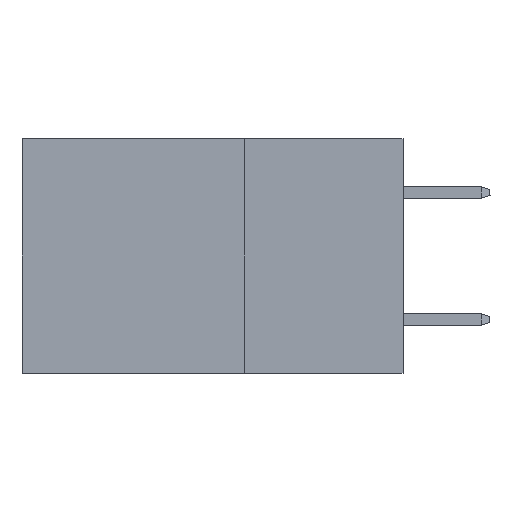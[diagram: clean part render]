
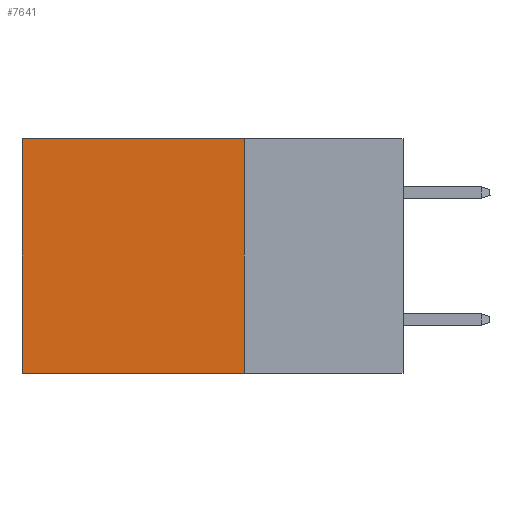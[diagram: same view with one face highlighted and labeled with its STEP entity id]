
A CAD part, left-side view. The second image highlights one B-rep face of the part: STEP entity #7641.
In plain terms, the highlighted planar face has unit normal (-1, 0, 0).
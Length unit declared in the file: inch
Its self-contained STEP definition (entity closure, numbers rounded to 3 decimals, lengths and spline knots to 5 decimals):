
#786 = DIRECTION ( 'NONE',  ( 1., 0., 0. ) ) ;
#1790 = CARTESIAN_POINT ( 'NONE',  ( 0.2875, 0.25, -0.37 ) ) ;
#4388 = DIRECTION ( 'NONE',  ( 0., 0., -1. ) ) ;
#4573 = DIRECTION ( 'NONE',  ( 0., 0., -1. ) ) ;
#4830 = CARTESIAN_POINT ( 'NONE',  ( 0.2875, 0.25, 0. ) ) ;
#6006 = ORIENTED_EDGE ( 'NONE', *, *, #22794, .F. ) ;
#7256 = VECTOR ( 'NONE', #27982, 39.37008 ) ;
#7554 = PLANE ( 'NONE',  #19619 ) ;
#7641 = ADVANCED_FACE ( 'NONE', ( #35799 ), #7554, .F. ) ;
#7996 = ORIENTED_EDGE ( 'NONE', *, *, #14541, .T. ) ;
#9535 = VECTOR ( 'NONE', #41426, 39.37008 ) ;
#10959 = CARTESIAN_POINT ( 'NONE',  ( 0.2875, 0.25, 0. ) ) ;
#13376 = CARTESIAN_POINT ( 'NONE',  ( 0.2875, 0.6, 0. ) ) ;
#14541 = EDGE_CURVE ( 'NONE', #29327, #15998, #15408, .T. ) ;
#15018 = VERTEX_POINT ( 'NONE', #1790 ) ;
#15116 = DIRECTION ( 'NONE',  ( 0., 0., -1. ) ) ;
#15408 = LINE ( 'NONE', #19041, #36087 ) ;
#15998 = VERTEX_POINT ( 'NONE', #42530 ) ;
#19041 = CARTESIAN_POINT ( 'NONE',  ( 0.2875, 0.6, 0. ) ) ;
#19619 = AXIS2_PLACEMENT_3D ( 'NONE', #4830, #786, #4388 ) ;
#21358 = LINE ( 'NONE', #27669, #9535 ) ;
#22794 = EDGE_CURVE ( 'NONE', #27226, #15018, #25311, .T. ) ;
#25311 = LINE ( 'NONE', #32509, #34199 ) ;
#27226 = VERTEX_POINT ( 'NONE', #10959 ) ;
#27669 = CARTESIAN_POINT ( 'NONE',  ( 0.2875, 0.25, -0.37 ) ) ;
#27982 = DIRECTION ( 'NONE',  ( 0., 1., 0. ) ) ;
#29327 = VERTEX_POINT ( 'NONE', #13376 ) ;
#30481 = CARTESIAN_POINT ( 'NONE',  ( 0.2875, 0.25, 0. ) ) ;
#32103 = EDGE_CURVE ( 'NONE', #27226, #29327, #44274, .T. ) ;
#32509 = CARTESIAN_POINT ( 'NONE',  ( 0.2875, 0.25, 0. ) ) ;
#34091 = EDGE_LOOP ( 'NONE', ( #7996, #34408, #6006, #35212 ) ) ;
#34199 = VECTOR ( 'NONE', #15116, 39.37008 ) ;
#34408 = ORIENTED_EDGE ( 'NONE', *, *, #34499, .F. ) ;
#34499 = EDGE_CURVE ( 'NONE', #15018, #15998, #21358, .T. ) ;
#35212 = ORIENTED_EDGE ( 'NONE', *, *, #32103, .T. ) ;
#35799 = FACE_OUTER_BOUND ( 'NONE', #34091, .T. ) ;
#36087 = VECTOR ( 'NONE', #4573, 39.37008 ) ;
#41426 = DIRECTION ( 'NONE',  ( 0., 1., 0. ) ) ;
#42530 = CARTESIAN_POINT ( 'NONE',  ( 0.2875, 0.6, -0.37 ) ) ;
#44274 = LINE ( 'NONE', #30481, #7256 ) ;
